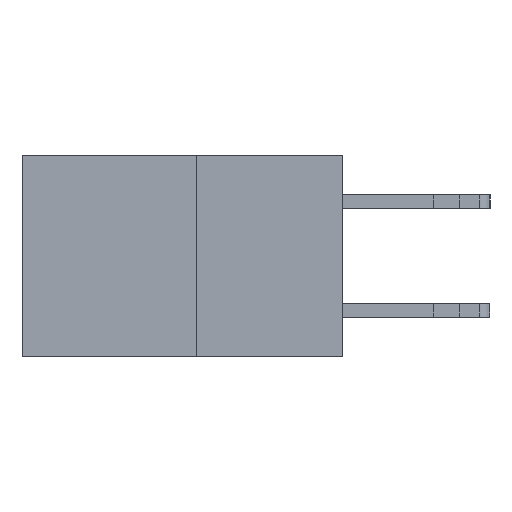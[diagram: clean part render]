
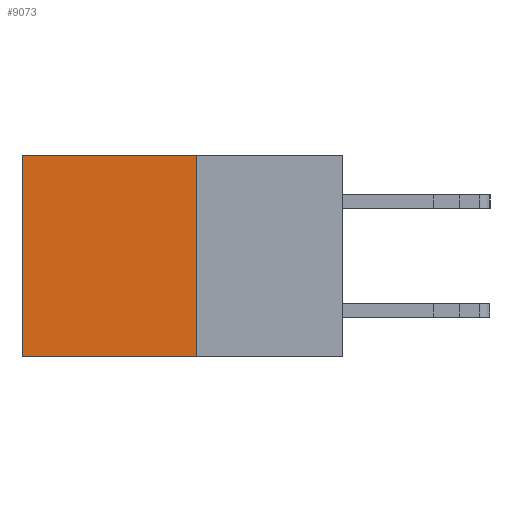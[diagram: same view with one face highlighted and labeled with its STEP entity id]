
A CAD part, left-side view. The second image highlights one B-rep face of the part: STEP entity #9073.
In plain terms, the highlighted planar face has unit normal (-1, 0, 0).
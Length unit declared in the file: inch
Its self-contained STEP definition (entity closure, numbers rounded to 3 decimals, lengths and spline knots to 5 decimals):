
#10 = VERTEX_POINT ( 'NONE', #8625 ) ;
#428 = ORIENTED_EDGE ( 'NONE', *, *, #5129, .T. ) ;
#618 = LINE ( 'NONE', #4313, #11570 ) ;
#792 = ORIENTED_EDGE ( 'NONE', *, *, #10552, .F. ) ;
#895 = VERTEX_POINT ( 'NONE', #10351 ) ;
#1144 = ORIENTED_EDGE ( 'NONE', *, *, #11169, .T. ) ;
#1240 = LINE ( 'NONE', #6197, #4518 ) ;
#1242 = DIRECTION ( 'NONE',  ( 1., 0., 0. ) ) ;
#1470 = VERTEX_POINT ( 'NONE', #2561 ) ;
#1884 = VERTEX_POINT ( 'NONE', #4760 ) ;
#2074 = VECTOR ( 'NONE', #6089, 39.37008 ) ;
#2145 = DIRECTION ( 'NONE',  ( 0., 0., -1. ) ) ;
#2561 = CARTESIAN_POINT ( 'NONE',  ( 0.277, 0.59, -0.37 ) ) ;
#3432 = LINE ( 'NONE', #4966, #2074 ) ;
#3709 = ORIENTED_EDGE ( 'NONE', *, *, #6789, .F. ) ;
#4272 = VECTOR ( 'NONE', #8683, 39.37008 ) ;
#4313 = CARTESIAN_POINT ( 'NONE',  ( 0.277, 0.27, -0.37 ) ) ;
#4518 = VECTOR ( 'NONE', #13767, 39.37008 ) ;
#4760 = CARTESIAN_POINT ( 'NONE',  ( 0.277, 0.59, 0. ) ) ;
#4948 = EDGE_LOOP ( 'NONE', ( #428, #792, #3709, #1144 ) ) ;
#4966 = CARTESIAN_POINT ( 'NONE',  ( 0.277, 0.27, 0. ) ) ;
#5129 = EDGE_CURVE ( 'NONE', #1884, #1470, #7527, .T. ) ;
#5655 = CARTESIAN_POINT ( 'NONE',  ( 0.277, 0.27, -0.37 ) ) ;
#6089 = DIRECTION ( 'NONE',  ( 0., 1., 0. ) ) ;
#6197 = CARTESIAN_POINT ( 'NONE',  ( 0.277, 0.27, -0.37 ) ) ;
#6731 = AXIS2_PLACEMENT_3D ( 'NONE', #5655, #1242, #8898 ) ;
#6789 = EDGE_CURVE ( 'NONE', #895, #10, #618, .T. ) ;
#7527 = LINE ( 'NONE', #14077, #4272 ) ;
#7806 = PLANE ( 'NONE',  #6731 ) ;
#8625 = CARTESIAN_POINT ( 'NONE',  ( 0.277, 0.27, -0.37 ) ) ;
#8683 = DIRECTION ( 'NONE',  ( 0., 0., -1. ) ) ;
#8898 = DIRECTION ( 'NONE',  ( 0., 0., -1. ) ) ;
#9073 = ADVANCED_FACE ( 'NONE', ( #13721 ), #7806, .F. ) ;
#10351 = CARTESIAN_POINT ( 'NONE',  ( 0.277, 0.27, 0. ) ) ;
#10552 = EDGE_CURVE ( 'NONE', #10, #1470, #1240, .T. ) ;
#11169 = EDGE_CURVE ( 'NONE', #895, #1884, #3432, .T. ) ;
#11570 = VECTOR ( 'NONE', #2145, 39.37008 ) ;
#13721 = FACE_OUTER_BOUND ( 'NONE', #4948, .T. ) ;
#13767 = DIRECTION ( 'NONE',  ( 0., 1., 0. ) ) ;
#14077 = CARTESIAN_POINT ( 'NONE',  ( 0.277, 0.59, -0.37 ) ) ;
